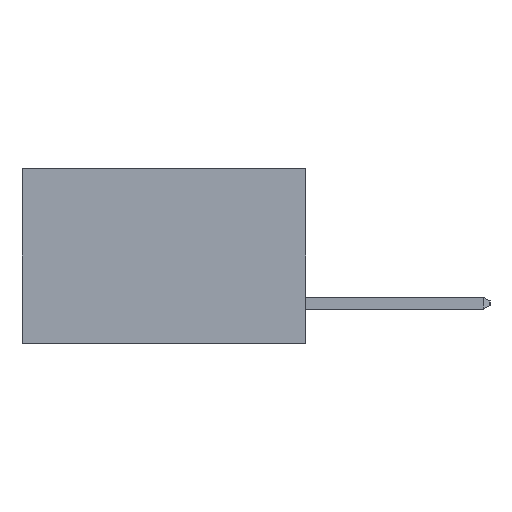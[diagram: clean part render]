
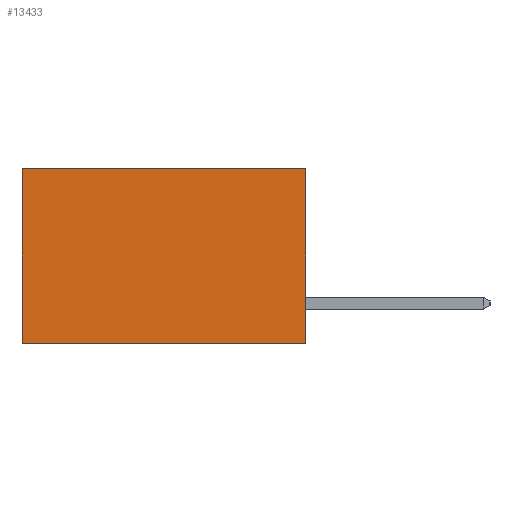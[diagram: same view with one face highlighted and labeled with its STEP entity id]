
A CAD part, left-side view. The second image highlights one B-rep face of the part: STEP entity #13433.
In plain terms, the highlighted planar face has unit normal (-1, 0, 0).
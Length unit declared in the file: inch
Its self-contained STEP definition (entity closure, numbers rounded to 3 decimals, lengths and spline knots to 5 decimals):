
#654 = CARTESIAN_POINT ( 'NONE',  ( 0.298, 0.6, -0.37 ) ) ;
#922 = ORIENTED_EDGE ( 'NONE', *, *, #19748, .T. ) ;
#2016 = AXIS2_PLACEMENT_3D ( 'NONE', #18455, #6272, #20467 ) ;
#2196 = PLANE ( 'NONE',  #2016 ) ;
#4255 = LINE ( 'NONE', #13976, #19806 ) ;
#6145 = EDGE_CURVE ( 'NONE', #19769, #22201, #25638, .T. ) ;
#6272 = DIRECTION ( 'NONE',  ( 1., 0., 0. ) ) ;
#6910 = ORIENTED_EDGE ( 'NONE', *, *, #16954, .F. ) ;
#8248 = VERTEX_POINT ( 'NONE', #17809 ) ;
#9491 = FACE_OUTER_BOUND ( 'NONE', #16152, .T. ) ;
#10289 = CARTESIAN_POINT ( 'NONE',  ( 0.298, 0., 0. ) ) ;
#10784 = DIRECTION ( 'NONE',  ( 0., 1., 0. ) ) ;
#12129 = CARTESIAN_POINT ( 'NONE',  ( 0.298, 0., -0.37 ) ) ;
#12155 = DIRECTION ( 'NONE',  ( 0., 0., -1. ) ) ;
#12381 = VECTOR ( 'NONE', #18276, 39.37008 ) ;
#13433 = ADVANCED_FACE ( 'NONE', ( #9491 ), #2196, .F. ) ;
#13730 = LINE ( 'NONE', #22221, #18560 ) ;
#13976 = CARTESIAN_POINT ( 'NONE',  ( 0.298, 0.6, 0. ) ) ;
#15043 = VECTOR ( 'NONE', #10784, 39.37008 ) ;
#16070 = DIRECTION ( 'NONE',  ( 0., 0., -1. ) ) ;
#16152 = EDGE_LOOP ( 'NONE', ( #922, #6910, #19109, #21070 ) ) ;
#16954 = EDGE_CURVE ( 'NONE', #8248, #17178, #17817, .T. ) ;
#17178 = VERTEX_POINT ( 'NONE', #654 ) ;
#17809 = CARTESIAN_POINT ( 'NONE',  ( 0.298, 0., -0.37 ) ) ;
#17817 = LINE ( 'NONE', #12129, #12381 ) ;
#18276 = DIRECTION ( 'NONE',  ( 0., 1., 0. ) ) ;
#18455 = CARTESIAN_POINT ( 'NONE',  ( 0.298, 0., 0. ) ) ;
#18560 = VECTOR ( 'NONE', #12155, 39.37008 ) ;
#19109 = ORIENTED_EDGE ( 'NONE', *, *, #19794, .F. ) ;
#19748 = EDGE_CURVE ( 'NONE', #22201, #17178, #4255, .T. ) ;
#19769 = VERTEX_POINT ( 'NONE', #22137 ) ;
#19794 = EDGE_CURVE ( 'NONE', #19769, #8248, #13730, .T. ) ;
#19806 = VECTOR ( 'NONE', #16070, 39.37008 ) ;
#20467 = DIRECTION ( 'NONE',  ( 0., 0., -1. ) ) ;
#21070 = ORIENTED_EDGE ( 'NONE', *, *, #6145, .T. ) ;
#22137 = CARTESIAN_POINT ( 'NONE',  ( 0.298, 0., 0. ) ) ;
#22201 = VERTEX_POINT ( 'NONE', #24914 ) ;
#22221 = CARTESIAN_POINT ( 'NONE',  ( 0.298, 0., 0. ) ) ;
#24914 = CARTESIAN_POINT ( 'NONE',  ( 0.298, 0.6, 0. ) ) ;
#25638 = LINE ( 'NONE', #10289, #15043 ) ;
